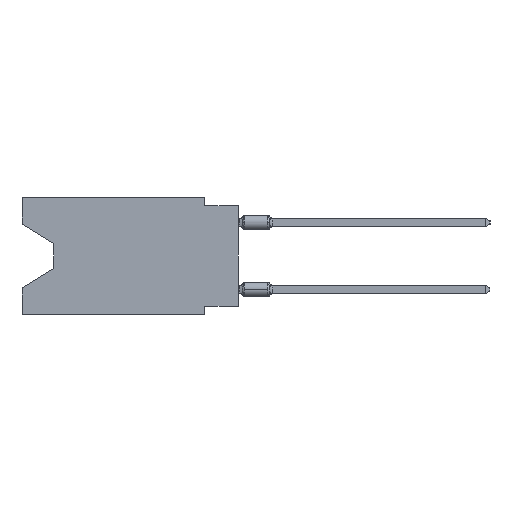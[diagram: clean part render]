
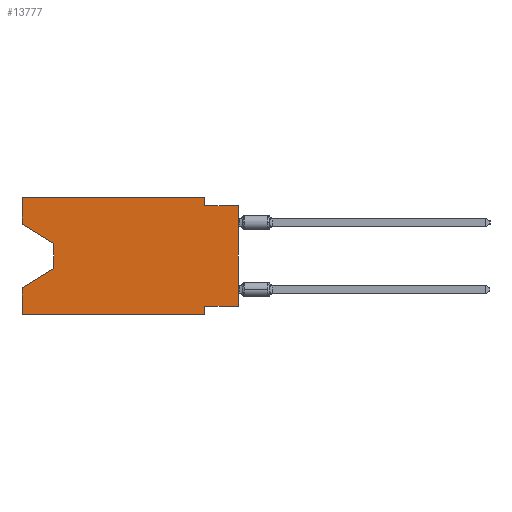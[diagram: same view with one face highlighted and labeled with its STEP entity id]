
A CAD part, left-side view. The second image highlights one B-rep face of the part: STEP entity #13777.
In plain terms, the highlighted planar face has unit normal (-1, 0, 0).
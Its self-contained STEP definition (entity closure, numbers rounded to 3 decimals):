
#1225 = CARTESIAN_POINT ( 'NONE',  ( 0., 16.383, -2.038 ) ) ;
#1310 = CARTESIAN_POINT ( 'NONE',  ( 0., 0., 0. ) ) ;
#3679 = CARTESIAN_POINT ( 'NONE',  ( 0., 2.54, -8.89 ) ) ;
#4029 = ORIENTED_EDGE ( 'NONE', *, *, #27857, .F. ) ;
#4901 = DIRECTION ( 'NONE',  ( 0., -1., 0. ) ) ;
#5063 = LINE ( 'NONE', #13652, #5370 ) ;
#5370 = VECTOR ( 'NONE', #44679, 1000. ) ;
#5617 = VERTEX_POINT ( 'NONE', #20927 ) ;
#5632 = DIRECTION ( 'NONE',  ( 0., -0.855, -0.519 ) ) ;
#6413 = CARTESIAN_POINT ( 'NONE',  ( 0., 0., -0.635 ) ) ;
#7048 = LINE ( 'NONE', #38084, #23679 ) ;
#7323 = CARTESIAN_POINT ( 'NONE',  ( 0., 2.54, 0. ) ) ;
#7600 = FACE_OUTER_BOUND ( 'NONE', #51335, .T. ) ;
#7949 = ORIENTED_EDGE ( 'NONE', *, *, #17125, .F. ) ;
#7977 = VECTOR ( 'NONE', #5632, 1000. ) ;
#8457 = VERTEX_POINT ( 'NONE', #34672 ) ;
#8824 = EDGE_CURVE ( 'NONE', #22177, #18025, #35591, .T. ) ;
#9002 = EDGE_CURVE ( 'NONE', #11749, #37362, #5063, .T. ) ;
#9041 = CARTESIAN_POINT ( 'NONE',  ( 0., 0., -0.635 ) ) ;
#10066 = EDGE_CURVE ( 'NONE', #15858, #39165, #13635, .T. ) ;
#10859 = CARTESIAN_POINT ( 'NONE',  ( 0., 16.383, -2.038 ) ) ;
#11749 = VERTEX_POINT ( 'NONE', #12801 ) ;
#11777 = DIRECTION ( 'NONE',  ( 1., 0., 0. ) ) ;
#11848 = VECTOR ( 'NONE', #31573, 1000. ) ;
#11972 = CARTESIAN_POINT ( 'NONE',  ( 0., 2.54, -8.89 ) ) ;
#12801 = CARTESIAN_POINT ( 'NONE',  ( 0., 13.97, -3.505 ) ) ;
#13635 = LINE ( 'NONE', #45432, #44616 ) ;
#13652 = CARTESIAN_POINT ( 'NONE',  ( 0., 13.97, -3.505 ) ) ;
#13777 = ADVANCED_FACE ( 'NONE', ( #7600 ), #23519, .F. ) ;
#14074 = VECTOR ( 'NONE', #16645, 1000. ) ;
#15265 = LINE ( 'NONE', #6413, #37168 ) ;
#15271 = ORIENTED_EDGE ( 'NONE', *, *, #21336, .F. ) ;
#15858 = VERTEX_POINT ( 'NONE', #10859 ) ;
#16195 = CARTESIAN_POINT ( 'NONE',  ( 0., 16.383, 0. ) ) ;
#16224 = VECTOR ( 'NONE', #17196, 1000. ) ;
#16645 = DIRECTION ( 'NONE',  ( 0., 0., -1. ) ) ;
#17125 = EDGE_CURVE ( 'NONE', #38743, #8457, #35952, .T. ) ;
#17196 = DIRECTION ( 'NONE',  ( 0., 0., 1. ) ) ;
#18025 = VERTEX_POINT ( 'NONE', #11972 ) ;
#20927 = CARTESIAN_POINT ( 'NONE',  ( 0., 0., -8.255 ) ) ;
#21104 = LINE ( 'NONE', #1310, #16224 ) ;
#21244 = VERTEX_POINT ( 'NONE', #33936 ) ;
#21336 = EDGE_CURVE ( 'NONE', #5617, #28658, #34439, .T. ) ;
#22177 = VERTEX_POINT ( 'NONE', #48908 ) ;
#23519 = PLANE ( 'NONE',  #38290 ) ;
#23679 = VECTOR ( 'NONE', #34945, 1000. ) ;
#24188 = ORIENTED_EDGE ( 'NONE', *, *, #31612, .T. ) ;
#24222 = CARTESIAN_POINT ( 'NONE',  ( 0., 2.54, 0. ) ) ;
#25871 = ORIENTED_EDGE ( 'NONE', *, *, #10066, .F. ) ;
#26317 = ORIENTED_EDGE ( 'NONE', *, *, #50021, .F. ) ;
#27234 = CARTESIAN_POINT ( 'NONE',  ( 0., 2.54, -8.255 ) ) ;
#27685 = DIRECTION ( 'NONE',  ( 0., 0., -1. ) ) ;
#27857 = EDGE_CURVE ( 'NONE', #39165, #38743, #37482, .T. ) ;
#28184 = LINE ( 'NONE', #3679, #11848 ) ;
#28384 = CARTESIAN_POINT ( 'NONE',  ( 0., 16.383, 0. ) ) ;
#28658 = VERTEX_POINT ( 'NONE', #27234 ) ;
#29961 = ORIENTED_EDGE ( 'NONE', *, *, #9002, .T. ) ;
#30374 = EDGE_CURVE ( 'NONE', #37362, #21244, #44838, .T. ) ;
#31163 = DIRECTION ( 'NONE',  ( 0., -1., 0. ) ) ;
#31416 = CARTESIAN_POINT ( 'NONE',  ( 0., 16.383, -8.89 ) ) ;
#31573 = DIRECTION ( 'NONE',  ( 0., 0., -1. ) ) ;
#31612 = EDGE_CURVE ( 'NONE', #5617, #43394, #21104, .T. ) ;
#32901 = CARTESIAN_POINT ( 'NONE',  ( 0., 13.97, -5.385 ) ) ;
#33049 = ORIENTED_EDGE ( 'NONE', *, *, #30374, .T. ) ;
#33704 = DIRECTION ( 'NONE',  ( 0., 0., 1. ) ) ;
#33936 = CARTESIAN_POINT ( 'NONE',  ( 0., 16.383, -6.852 ) ) ;
#34439 = LINE ( 'NONE', #46166, #40492 ) ;
#34672 = CARTESIAN_POINT ( 'NONE',  ( 0., 2.54, -0.635 ) ) ;
#34687 = ORIENTED_EDGE ( 'NONE', *, *, #47559, .F. ) ;
#34945 = DIRECTION ( 'NONE',  ( 0., 0., 1. ) ) ;
#35591 = LINE ( 'NONE', #31416, #41184 ) ;
#35952 = LINE ( 'NONE', #24222, #14074 ) ;
#36924 = LINE ( 'NONE', #1225, #7977 ) ;
#37168 = VECTOR ( 'NONE', #31163, 1000. ) ;
#37362 = VERTEX_POINT ( 'NONE', #32901 ) ;
#37482 = LINE ( 'NONE', #28384, #42259 ) ;
#38084 = CARTESIAN_POINT ( 'NONE',  ( 0., 16.383, 0. ) ) ;
#38287 = CARTESIAN_POINT ( 'NONE',  ( 0., 16.383, 0. ) ) ;
#38290 = AXIS2_PLACEMENT_3D ( 'NONE', #16195, #11777, #27685 ) ;
#38743 = VERTEX_POINT ( 'NONE', #7323 ) ;
#39165 = VERTEX_POINT ( 'NONE', #38287 ) ;
#39458 = EDGE_CURVE ( 'NONE', #22177, #21244, #7048, .T. ) ;
#40269 = DIRECTION ( 'NONE',  ( 0., -1., 0. ) ) ;
#40492 = VECTOR ( 'NONE', #49339, 1000. ) ;
#41184 = VECTOR ( 'NONE', #40269, 1000. ) ;
#42259 = VECTOR ( 'NONE', #4901, 1000. ) ;
#43152 = ORIENTED_EDGE ( 'NONE', *, *, #39458, .F. ) ;
#43394 = VERTEX_POINT ( 'NONE', #9041 ) ;
#44616 = VECTOR ( 'NONE', #33704, 1000. ) ;
#44679 = DIRECTION ( 'NONE',  ( 0., 0., -1. ) ) ;
#44838 = LINE ( 'NONE', #49531, #45750 ) ;
#45432 = CARTESIAN_POINT ( 'NONE',  ( 0., 16.383, 0. ) ) ;
#45750 = VECTOR ( 'NONE', #48761, 1000. ) ;
#46166 = CARTESIAN_POINT ( 'NONE',  ( 0., 0., -8.255 ) ) ;
#47053 = EDGE_CURVE ( 'NONE', #15858, #11749, #36924, .T. ) ;
#47559 = EDGE_CURVE ( 'NONE', #8457, #43394, #15265, .T. ) ;
#48396 = ORIENTED_EDGE ( 'NONE', *, *, #8824, .T. ) ;
#48695 = ORIENTED_EDGE ( 'NONE', *, *, #47053, .T. ) ;
#48761 = DIRECTION ( 'NONE',  ( 0., 0.855, -0.519 ) ) ;
#48908 = CARTESIAN_POINT ( 'NONE',  ( 0., 16.383, -8.89 ) ) ;
#49339 = DIRECTION ( 'NONE',  ( 0., 1., 0. ) ) ;
#49531 = CARTESIAN_POINT ( 'NONE',  ( 0., 13.97, -5.385 ) ) ;
#50021 = EDGE_CURVE ( 'NONE', #28658, #18025, #28184, .T. ) ;
#51335 = EDGE_LOOP ( 'NONE', ( #48695, #29961, #33049, #43152, #48396, #26317, #15271, #24188, #34687, #7949, #4029, #25871 ) ) ;
